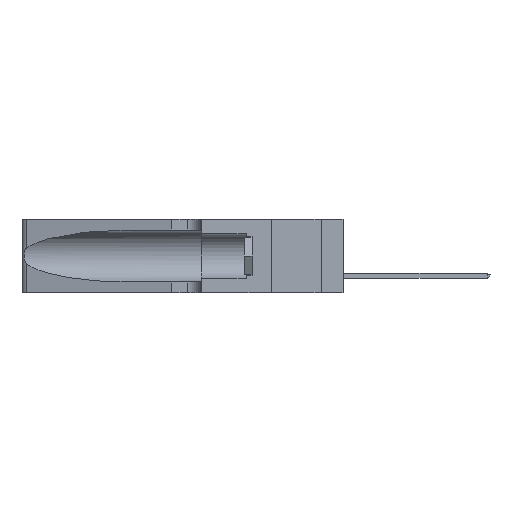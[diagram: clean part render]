
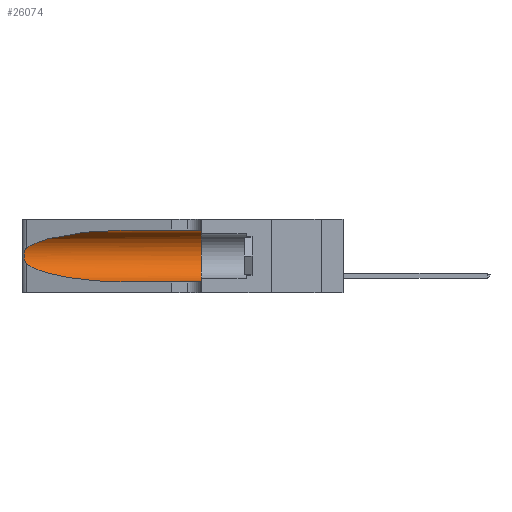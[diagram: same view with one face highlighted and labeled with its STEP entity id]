
A CAD part, left-side view. The second image highlights one B-rep face of the part: STEP entity #26074.
In plain terms, the highlighted cylindrical face has radius 3.308 mm (diameter 6.617 mm), a partial arc.
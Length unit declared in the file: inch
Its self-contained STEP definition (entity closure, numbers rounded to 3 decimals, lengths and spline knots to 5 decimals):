
#270 = ORIENTED_EDGE ( 'NONE', *, *, #5570, .T. ) ;
#397 = LINE ( 'NONE', #12870, #23389 ) ;
#544 = DIRECTION ( 'NONE',  ( 0., -1., 0. ) ) ;
#969 =( BOUNDED_CURVE ( )  B_SPLINE_CURVE ( 3, ( #33063, #27698, #2765, #30009 ),
 .UNSPECIFIED., .F., .F. ) 
 B_SPLINE_CURVE_WITH_KNOTS ( ( 4, 4 ),
 ( 3.44316, 4.71239 ),
 .UNSPECIFIED. ) 
 CURVE ( )  GEOMETRIC_REPRESENTATION_ITEM ( )  RATIONAL_B_SPLINE_CURVE ( ( 1., 0.87, 0.87, 1. ) ) 
 REPRESENTATION_ITEM ( '' )  );
#1381 = CARTESIAN_POINT ( 'NONE',  ( 0.25487, 1.22718, 0.22369 ) ) ;
#1630 = EDGE_LOOP ( 'NONE', ( #11090, #34688, #270, #7457, #21264, #33792 ) ) ;
#2765 = CARTESIAN_POINT ( 'NONE',  ( 0.18966, 0.96281, 0.05475 ) ) ;
#3243 = CARTESIAN_POINT ( 'NONE',  ( 0.25487, 1.22718, 0.14631 ) ) ;
#4009 = CARTESIAN_POINT ( 'NONE',  ( 0.1305, 1.61858, 0.31525 ) ) ;
#4900 = DIRECTION ( 'NONE',  ( 0., -1., 0. ) ) ;
#5570 = EDGE_CURVE ( 'NONE', #19233, #26484, #969, .T. ) ;
#6231 = VERTEX_POINT ( 'NONE', #11357 ) ;
#6990 = DIRECTION ( 'NONE',  ( 0., 1., 0. ) ) ;
#7295 = CARTESIAN_POINT ( 'NONE',  ( 0.1305, 0.72297, 0.05475 ) ) ;
#7457 = ORIENTED_EDGE ( 'NONE', *, *, #23147, .T. ) ;
#7597 = AXIS2_PLACEMENT_3D ( 'NONE', #32411, #4900, #15861 ) ;
#7720 = VERTEX_POINT ( 'NONE', #35156 ) ;
#7910 = CARTESIAN_POINT ( 'NONE',  ( 0.25639, 1.23184, 0.21858 ) ) ;
#8479 = B_SPLINE_CURVE_WITH_KNOTS ( 'NONE', 3,
 ( #21697, #24472, #7910, #10099, #35536, #10665, #30369, #33103, #22130, #16316, #19571, #33553, #31051, #3243 ),
 .UNSPECIFIED., .F., .F.,
 ( 4, 2, 2, 2, 2, 2, 4 ),
 ( 0., 0.00027, 0.00053, 0.00107, 0.0016, 0.00187, 0.00214 ),
 .UNSPECIFIED. ) ;
#9108 = CARTESIAN_POINT ( 'NONE',  ( 0.1305, 0.35, 0.185 ) ) ;
#10099 = CARTESIAN_POINT ( 'NONE',  ( 0.25787, 1.23484, 0.2124 ) ) ;
#10665 = CARTESIAN_POINT ( 'NONE',  ( 0.26018, 1.23835, 0.19895 ) ) ;
#11090 = ORIENTED_EDGE ( 'NONE', *, *, #11520, .T. ) ;
#11357 = CARTESIAN_POINT ( 'NONE',  ( 0.1305, 0.35, 0.31525 ) ) ;
#11520 = EDGE_CURVE ( 'NONE', #7720, #19597, #27805, .T. ) ;
#12870 = CARTESIAN_POINT ( 'NONE',  ( 0.1305, 1.61858, 0.05475 ) ) ;
#13043 = CARTESIAN_POINT ( 'NONE',  ( 0.1305, 0.72297, 0.31525 ) ) ;
#13234 = FACE_OUTER_BOUND ( 'NONE', #1630, .T. ) ;
#13545 = EDGE_CURVE ( 'NONE', #19597, #19233, #8479, .T. ) ;
#14206 = VERTEX_POINT ( 'NONE', #17222 ) ;
#15861 = DIRECTION ( 'NONE',  ( 0., 0., -1. ) ) ;
#15882 = AXIS2_PLACEMENT_3D ( 'NONE', #9108, #6990, #33741 ) ;
#16316 = CARTESIAN_POINT ( 'NONE',  ( 0.25856, 1.23593, 0.16098 ) ) ;
#16411 = VECTOR ( 'NONE', #20682, 39.37008 ) ;
#17222 = CARTESIAN_POINT ( 'NONE',  ( 0.1305, 0.35, 0.05475 ) ) ;
#18787 = CARTESIAN_POINT ( 'NONE',  ( 0.25487, 1.22718, 0.14631 ) ) ;
#19039 = LINE ( 'NONE', #4009, #16411 ) ;
#19233 = VERTEX_POINT ( 'NONE', #18787 ) ;
#19571 = CARTESIAN_POINT ( 'NONE',  ( 0.25789, 1.23486, 0.15765 ) ) ;
#19597 = VERTEX_POINT ( 'NONE', #1381 ) ;
#20682 = DIRECTION ( 'NONE',  ( 0., -1., 0. ) ) ;
#21264 = ORIENTED_EDGE ( 'NONE', *, *, #25166, .F. ) ;
#21408 = CARTESIAN_POINT ( 'NONE',  ( 0.2373, 1.15595, 0.28018 ) ) ;
#21697 = CARTESIAN_POINT ( 'NONE',  ( 0.25487, 1.22718, 0.22369 ) ) ;
#22130 = CARTESIAN_POINT ( 'NONE',  ( 0.26017, 1.23833, 0.17102 ) ) ;
#23147 = EDGE_CURVE ( 'NONE', #26484, #14206, #397, .T. ) ;
#23389 = VECTOR ( 'NONE', #544, 39.37008 ) ;
#23677 = CIRCLE ( 'NONE', #15882, 0.13025 ) ;
#24472 = CARTESIAN_POINT ( 'NONE',  ( 0.25555, 1.22994, 0.2215 ) ) ;
#25166 = EDGE_CURVE ( 'NONE', #6231, #14206, #23677, .T. ) ;
#26074 = ADVANCED_FACE ( 'NONE', ( #13234 ), #33089, .F. ) ;
#26484 = VERTEX_POINT ( 'NONE', #7295 ) ;
#27222 = CARTESIAN_POINT ( 'NONE',  ( 0.25487, 1.22718, 0.22369 ) ) ;
#27438 = CARTESIAN_POINT ( 'NONE',  ( 0.18966, 0.96281, 0.31525 ) ) ;
#27698 = CARTESIAN_POINT ( 'NONE',  ( 0.2373, 1.15595, 0.08982 ) ) ;
#27805 =( BOUNDED_CURVE ( )  B_SPLINE_CURVE ( 3, ( #13043, #27438, #21408, #27222 ),
 .UNSPECIFIED., .F., .F. ) 
 B_SPLINE_CURVE_WITH_KNOTS ( ( 4, 4 ),
 ( 1.5708, 2.84003 ),
 .UNSPECIFIED. ) 
 CURVE ( )  GEOMETRIC_REPRESENTATION_ITEM ( )  RATIONAL_B_SPLINE_CURVE ( ( 1., 0.87, 0.87, 1. ) ) 
 REPRESENTATION_ITEM ( '' )  );
#30009 = CARTESIAN_POINT ( 'NONE',  ( 0.1305, 0.72297, 0.05475 ) ) ;
#30123 = EDGE_CURVE ( 'NONE', #7720, #6231, #19039, .T. ) ;
#30369 = CARTESIAN_POINT ( 'NONE',  ( 0.26075, 1.23896, 0.19203 ) ) ;
#31051 = CARTESIAN_POINT ( 'NONE',  ( 0.25555, 1.22993, 0.14849 ) ) ;
#32411 = CARTESIAN_POINT ( 'NONE',  ( 0.1305, 1.61858, 0.185 ) ) ;
#33063 = CARTESIAN_POINT ( 'NONE',  ( 0.25487, 1.22718, 0.14631 ) ) ;
#33089 = CYLINDRICAL_SURFACE ( 'NONE', #7597, 0.13025 ) ;
#33103 = CARTESIAN_POINT ( 'NONE',  ( 0.26075, 1.23896, 0.178 ) ) ;
#33553 = CARTESIAN_POINT ( 'NONE',  ( 0.25639, 1.23186, 0.15144 ) ) ;
#33741 = DIRECTION ( 'NONE',  ( 0., 0., 1. ) ) ;
#33792 = ORIENTED_EDGE ( 'NONE', *, *, #30123, .F. ) ;
#34688 = ORIENTED_EDGE ( 'NONE', *, *, #13545, .T. ) ;
#35156 = CARTESIAN_POINT ( 'NONE',  ( 0.1305, 0.72297, 0.31525 ) ) ;
#35536 = CARTESIAN_POINT ( 'NONE',  ( 0.25854, 1.2359, 0.20912 ) ) ;
